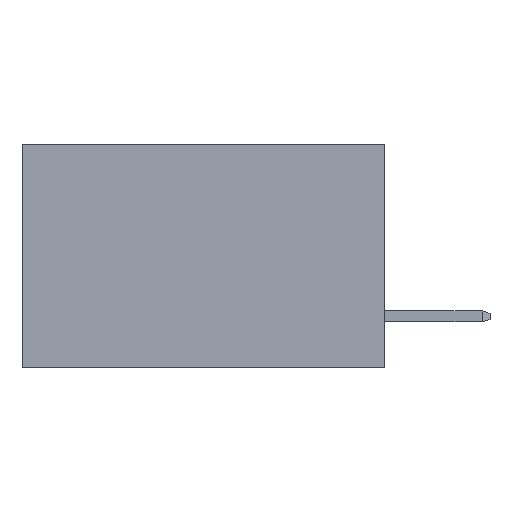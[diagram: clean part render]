
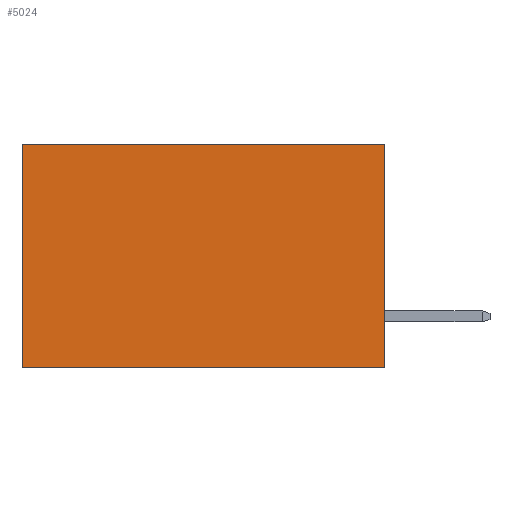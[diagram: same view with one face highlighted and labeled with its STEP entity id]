
A CAD part, left-side view. The second image highlights one B-rep face of the part: STEP entity #5024.
In plain terms, the highlighted planar face has unit normal (-1, 0, 0).
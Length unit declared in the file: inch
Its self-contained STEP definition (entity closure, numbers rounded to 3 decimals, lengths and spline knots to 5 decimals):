
#145 = CARTESIAN_POINT ( 'NONE',  ( 0.298, 0., 0. ) ) ;
#657 = EDGE_CURVE ( 'NONE', #10502, #17315, #11619, .T. ) ;
#1129 = CARTESIAN_POINT ( 'NONE',  ( 0.298, 0., 0. ) ) ;
#1956 = ORIENTED_EDGE ( 'NONE', *, *, #21292, .F. ) ;
#2674 = VECTOR ( 'NONE', #5100, 39.37008 ) ;
#3728 = CARTESIAN_POINT ( 'NONE',  ( 0.298, 0.6, 0. ) ) ;
#3811 = VECTOR ( 'NONE', #12543, 39.37008 ) ;
#4588 = EDGE_LOOP ( 'NONE', ( #11869, #1956, #5336, #16373 ) ) ;
#4598 = DIRECTION ( 'NONE',  ( 0., 1., 0. ) ) ;
#5024 = ADVANCED_FACE ( 'NONE', ( #15763 ), #20797, .F. ) ;
#5100 = DIRECTION ( 'NONE',  ( 0., 0., -1. ) ) ;
#5336 = ORIENTED_EDGE ( 'NONE', *, *, #7575, .F. ) ;
#6438 = CARTESIAN_POINT ( 'NONE',  ( 0.298, 0., -0.37 ) ) ;
#6761 = VECTOR ( 'NONE', #4598, 39.37008 ) ;
#7341 = VERTEX_POINT ( 'NONE', #6438 ) ;
#7575 = EDGE_CURVE ( 'NONE', #10502, #7341, #9547, .T. ) ;
#8807 = CARTESIAN_POINT ( 'NONE',  ( 0.298, 0.6, 0. ) ) ;
#8815 = CARTESIAN_POINT ( 'NONE',  ( 0.298, 0., 0. ) ) ;
#9547 = LINE ( 'NONE', #19787, #13723 ) ;
#10502 = VERTEX_POINT ( 'NONE', #145 ) ;
#11619 = LINE ( 'NONE', #1129, #6761 ) ;
#11869 = ORIENTED_EDGE ( 'NONE', *, *, #14125, .T. ) ;
#12543 = DIRECTION ( 'NONE',  ( 0., 1., 0. ) ) ;
#13506 = LINE ( 'NONE', #8807, #2674 ) ;
#13723 = VECTOR ( 'NONE', #15499, 39.37008 ) ;
#14125 = EDGE_CURVE ( 'NONE', #17315, #20051, #13506, .T. ) ;
#15499 = DIRECTION ( 'NONE',  ( 0., 0., -1. ) ) ;
#15763 = FACE_OUTER_BOUND ( 'NONE', #4588, .T. ) ;
#16035 = CARTESIAN_POINT ( 'NONE',  ( 0.298, 0.6, -0.37 ) ) ;
#16373 = ORIENTED_EDGE ( 'NONE', *, *, #657, .T. ) ;
#17315 = VERTEX_POINT ( 'NONE', #3728 ) ;
#19787 = CARTESIAN_POINT ( 'NONE',  ( 0.298, 0., 0. ) ) ;
#19953 = DIRECTION ( 'NONE',  ( 0., 0., -1. ) ) ;
#20051 = VERTEX_POINT ( 'NONE', #16035 ) ;
#20285 = AXIS2_PLACEMENT_3D ( 'NONE', #8815, #22765, #19953 ) ;
#20797 = PLANE ( 'NONE',  #20285 ) ;
#21292 = EDGE_CURVE ( 'NONE', #7341, #20051, #22027, .T. ) ;
#22027 = LINE ( 'NONE', #22775, #3811 ) ;
#22765 = DIRECTION ( 'NONE',  ( 1., 0., 0. ) ) ;
#22775 = CARTESIAN_POINT ( 'NONE',  ( 0.298, 0., -0.37 ) ) ;
